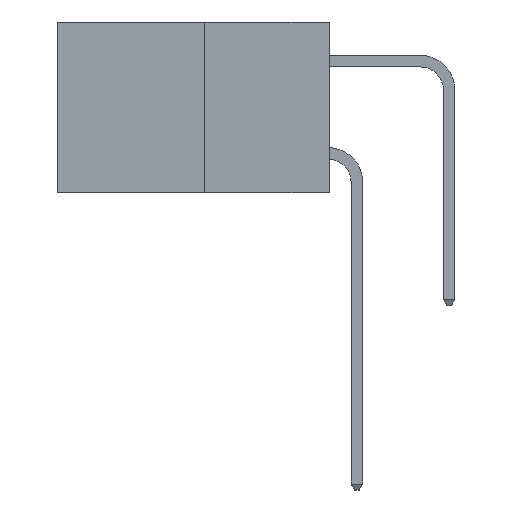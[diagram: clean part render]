
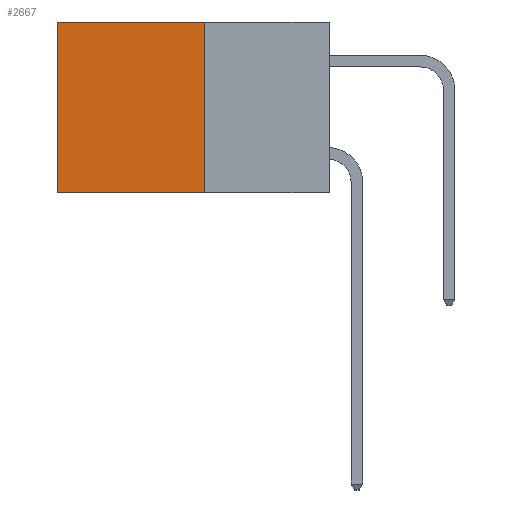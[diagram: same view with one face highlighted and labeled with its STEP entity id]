
A CAD part, left-side view. The second image highlights one B-rep face of the part: STEP entity #2667.
In plain terms, the highlighted planar face has unit normal (-1, 0, 0).
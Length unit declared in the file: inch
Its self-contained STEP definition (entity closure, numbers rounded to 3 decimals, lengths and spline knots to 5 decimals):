
#140 = PLANE ( 'NONE',  #7402 ) ;
#399 = CARTESIAN_POINT ( 'NONE',  ( 0.277, 0.59, -0.37 ) ) ;
#1474 = EDGE_CURVE ( 'NONE', #1722, #7937, #7820, .T. ) ;
#1722 = VERTEX_POINT ( 'NONE', #5172 ) ;
#1869 = DIRECTION ( 'NONE',  ( 0., 0., -1. ) ) ;
#1949 = CARTESIAN_POINT ( 'NONE',  ( 0.277, 0.59, -0.37 ) ) ;
#1989 = LINE ( 'NONE', #2161, #3917 ) ;
#2046 = DIRECTION ( 'NONE',  ( 0., 1., 0. ) ) ;
#2161 = CARTESIAN_POINT ( 'NONE',  ( 0.277, 0.27, -0.37 ) ) ;
#2667 = ADVANCED_FACE ( 'NONE', ( #4337 ), #140, .F. ) ;
#3593 = VECTOR ( 'NONE', #8926, 39.37008 ) ;
#3886 = VECTOR ( 'NONE', #1869, 39.37008 ) ;
#3898 = VECTOR ( 'NONE', #5638, 39.37008 ) ;
#3917 = VECTOR ( 'NONE', #2046, 39.37008 ) ;
#4110 = EDGE_CURVE ( 'NONE', #8039, #7264, #7526, .T. ) ;
#4337 = FACE_OUTER_BOUND ( 'NONE', #6240, .T. ) ;
#5113 = EDGE_CURVE ( 'NONE', #7264, #7937, #1989, .T. ) ;
#5172 = CARTESIAN_POINT ( 'NONE',  ( 0.277, 0.59, 0. ) ) ;
#5638 = DIRECTION ( 'NONE',  ( 0., 1., 0. ) ) ;
#5877 = CARTESIAN_POINT ( 'NONE',  ( 0.277, 0.27, 0. ) ) ;
#5975 = EDGE_CURVE ( 'NONE', #8039, #1722, #9517, .T. ) ;
#6240 = EDGE_LOOP ( 'NONE', ( #6796, #6492, #6565, #6640 ) ) ;
#6492 = ORIENTED_EDGE ( 'NONE', *, *, #5113, .F. ) ;
#6565 = ORIENTED_EDGE ( 'NONE', *, *, #4110, .F. ) ;
#6640 = ORIENTED_EDGE ( 'NONE', *, *, #5975, .T. ) ;
#6742 = CARTESIAN_POINT ( 'NONE',  ( 0.277, 0.27, -0.37 ) ) ;
#6796 = ORIENTED_EDGE ( 'NONE', *, *, #1474, .T. ) ;
#7264 = VERTEX_POINT ( 'NONE', #9449 ) ;
#7299 = DIRECTION ( 'NONE',  ( 0., 0., -1. ) ) ;
#7308 = DIRECTION ( 'NONE',  ( 1., 0., 0. ) ) ;
#7402 = AXIS2_PLACEMENT_3D ( 'NONE', #6742, #7308, #7299 ) ;
#7526 = LINE ( 'NONE', #9067, #3593 ) ;
#7820 = LINE ( 'NONE', #1949, #3886 ) ;
#7937 = VERTEX_POINT ( 'NONE', #399 ) ;
#8039 = VERTEX_POINT ( 'NONE', #8197 ) ;
#8197 = CARTESIAN_POINT ( 'NONE',  ( 0.277, 0.27, 0. ) ) ;
#8926 = DIRECTION ( 'NONE',  ( 0., 0., -1. ) ) ;
#9067 = CARTESIAN_POINT ( 'NONE',  ( 0.277, 0.27, -0.37 ) ) ;
#9449 = CARTESIAN_POINT ( 'NONE',  ( 0.277, 0.27, -0.37 ) ) ;
#9517 = LINE ( 'NONE', #5877, #3898 ) ;
